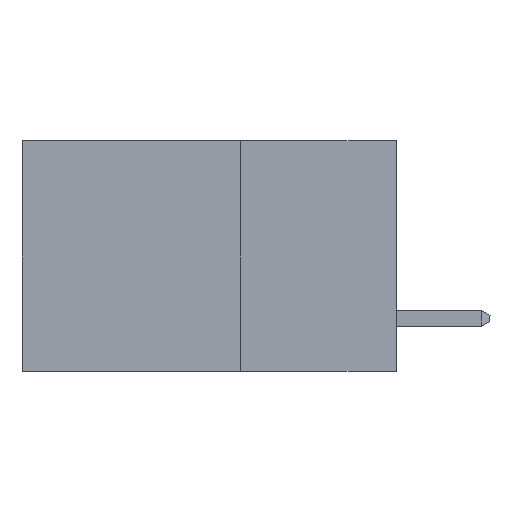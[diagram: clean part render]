
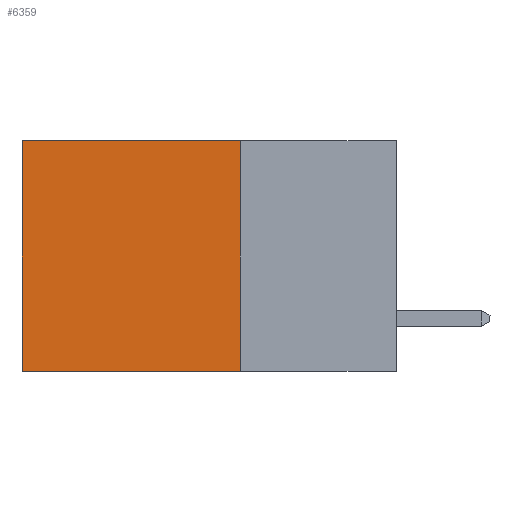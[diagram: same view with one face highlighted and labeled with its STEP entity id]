
A CAD part, left-side view. The second image highlights one B-rep face of the part: STEP entity #6359.
In plain terms, the highlighted planar face has unit normal (-1, 0, 0).
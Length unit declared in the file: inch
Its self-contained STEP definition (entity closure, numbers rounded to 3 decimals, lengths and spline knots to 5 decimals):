
#134 = VECTOR ( 'NONE', #7223, 39.37008 ) ;
#233 = CARTESIAN_POINT ( 'NONE',  ( 0.2615, 0.6, -0.37 ) ) ;
#275 = ORIENTED_EDGE ( 'NONE', *, *, #3447, .T. ) ;
#643 = VERTEX_POINT ( 'NONE', #233 ) ;
#1444 = EDGE_CURVE ( 'NONE', #6066, #6519, #1903, .T. ) ;
#1903 = LINE ( 'NONE', #6468, #134 ) ;
#1961 = CARTESIAN_POINT ( 'NONE',  ( 0.2615, 0.25, -0.37 ) ) ;
#2344 = VECTOR ( 'NONE', #7253, 39.37008 ) ;
#2401 = DIRECTION ( 'NONE',  ( 0., 1., 0. ) ) ;
#2433 = CARTESIAN_POINT ( 'NONE',  ( 0.2615, 0.25, -0.37 ) ) ;
#2492 = DIRECTION ( 'NONE',  ( 0., 1., 0. ) ) ;
#2554 = CARTESIAN_POINT ( 'NONE',  ( 0.2615, 0.25, 0. ) ) ;
#2664 = DIRECTION ( 'NONE',  ( 0., 0., -1. ) ) ;
#2672 = DIRECTION ( 'NONE',  ( 1., 0., 0. ) ) ;
#2683 = VECTOR ( 'NONE', #2492, 39.37008 ) ;
#2710 = CARTESIAN_POINT ( 'NONE',  ( 0.2615, 0.25, -0.37 ) ) ;
#2711 = PLANE ( 'NONE',  #6502 ) ;
#3156 = ORIENTED_EDGE ( 'NONE', *, *, #6421, .F. ) ;
#3359 = ORIENTED_EDGE ( 'NONE', *, *, #6384, .T. ) ;
#3447 = EDGE_CURVE ( 'NONE', #5800, #643, #4319, .T. ) ;
#4232 = VECTOR ( 'NONE', #2401, 39.37008 ) ;
#4319 = LINE ( 'NONE', #5677, #2344 ) ;
#4339 = CARTESIAN_POINT ( 'NONE',  ( 0.2615, 0.25, 0. ) ) ;
#4648 = LINE ( 'NONE', #2433, #4232 ) ;
#5080 = EDGE_LOOP ( 'NONE', ( #275, #3156, #6422, #3359 ) ) ;
#5677 = CARTESIAN_POINT ( 'NONE',  ( 0.2615, 0.6, -0.37 ) ) ;
#5800 = VERTEX_POINT ( 'NONE', #5847 ) ;
#5847 = CARTESIAN_POINT ( 'NONE',  ( 0.2615, 0.6, 0. ) ) ;
#6066 = VERTEX_POINT ( 'NONE', #4339 ) ;
#6348 = FACE_OUTER_BOUND ( 'NONE', #5080, .T. ) ;
#6359 = ADVANCED_FACE ( 'NONE', ( #6348 ), #2711, .F. ) ;
#6384 = EDGE_CURVE ( 'NONE', #6066, #5800, #7791, .T. ) ;
#6421 = EDGE_CURVE ( 'NONE', #6519, #643, #4648, .T. ) ;
#6422 = ORIENTED_EDGE ( 'NONE', *, *, #1444, .F. ) ;
#6468 = CARTESIAN_POINT ( 'NONE',  ( 0.2615, 0.25, -0.37 ) ) ;
#6502 = AXIS2_PLACEMENT_3D ( 'NONE', #2710, #2672, #2664 ) ;
#6519 = VERTEX_POINT ( 'NONE', #1961 ) ;
#7223 = DIRECTION ( 'NONE',  ( 0., 0., -1. ) ) ;
#7253 = DIRECTION ( 'NONE',  ( 0., 0., -1. ) ) ;
#7791 = LINE ( 'NONE', #2554, #2683 ) ;
